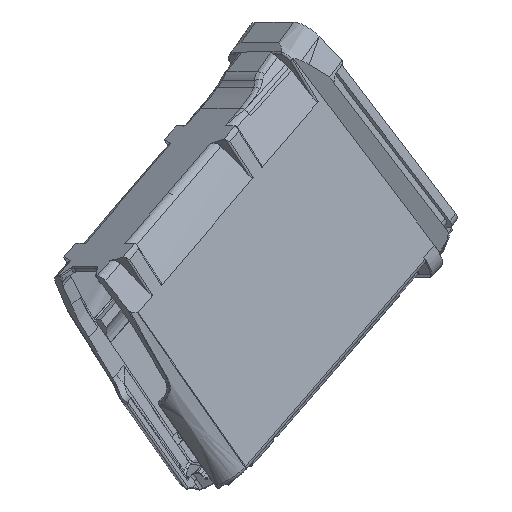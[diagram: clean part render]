
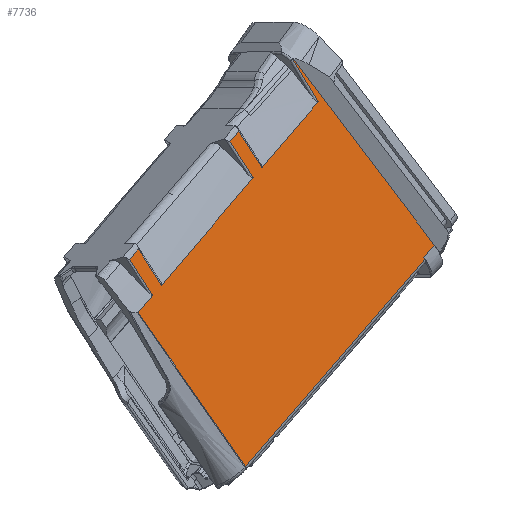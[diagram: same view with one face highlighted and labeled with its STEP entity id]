
A CAD part, top view. The second image highlights one B-rep face of the part: STEP entity #7736.
In plain terms, the highlighted face is planar.
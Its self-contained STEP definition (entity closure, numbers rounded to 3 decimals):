
#90 = EDGE_CURVE ( 'NONE', #14486, #7522, #11005, .T. ) ;
#168 = ORIENTED_EDGE ( 'NONE', *, *, #10661, .F. ) ;
#530 = VERTEX_POINT ( 'NONE', #7717 ) ;
#816 = ORIENTED_EDGE ( 'NONE', *, *, #90, .T. ) ;
#1443 = EDGE_CURVE ( 'NONE', #23993, #14486, #10864, .T. ) ;
#1557 = ORIENTED_EDGE ( 'NONE', *, *, #4731, .F. ) ;
#1852 = VERTEX_POINT ( 'NONE', #3733 ) ;
#2073 = EDGE_CURVE ( 'NONE', #16936, #530, #20423, .T. ) ;
#2199 = ORIENTED_EDGE ( 'NONE', *, *, #11765, .T. ) ;
#2383 = CARTESIAN_POINT ( 'NONE',  ( -29.284, 11.2, 43.909 ) ) ;
#2673 = EDGE_CURVE ( 'NONE', #12823, #11737, #12786, .T. ) ;
#2910 = VECTOR ( 'NONE', #3819, 1000. ) ;
#3134 = ORIENTED_EDGE ( 'NONE', *, *, #4787, .T. ) ;
#3635 = DIRECTION ( 'NONE',  ( -0.766, 0., 0.642 ) ) ;
#3688 = VERTEX_POINT ( 'NONE', #2383 ) ;
#3733 = CARTESIAN_POINT ( 'NONE',  ( 53.633, 11.2, 65.443 ) ) ;
#3819 = DIRECTION ( 'NONE',  ( -0.766, 0., 0.642 ) ) ;
#4002 = CARTESIAN_POINT ( 'NONE',  ( 6.541, 11.2, 99.837 ) ) ;
#4016 = CARTESIAN_POINT ( 'NONE',  ( 18.562, 11.2, 85.202 ) ) ;
#4152 = DIRECTION ( 'NONE',  ( -0.766, 0., 0.642 ) ) ;
#4637 = DIRECTION ( 'NONE',  ( -0.732, 0., -0.682 ) ) ;
#4731 = EDGE_CURVE ( 'NONE', #7395, #26562, #22648, .T. ) ;
#4787 = EDGE_CURVE ( 'NONE', #10811, #17255, #15645, .T. ) ;
#5304 = VECTOR ( 'NONE', #20542, 1000. ) ;
#5463 = DIRECTION ( 'NONE',  ( -0.664, 0., -0.748 ) ) ;
#6243 = CARTESIAN_POINT ( 'NONE',  ( -28.739, 11.2, 60.549 ) ) ;
#6341 = LINE ( 'NONE', #12766, #2910 ) ;
#6432 = DIRECTION ( 'NONE',  ( 0.642, 0., 0.766 ) ) ;
#7179 = DIRECTION ( 'NONE',  ( 0.668, 0., 0.744 ) ) ;
#7395 = VERTEX_POINT ( 'NONE', #25518 ) ;
#7498 = CARTESIAN_POINT ( 'NONE',  ( -28.949, 11.2, 44.282 ) ) ;
#7522 = VERTEX_POINT ( 'NONE', #4002 ) ;
#7529 = ORIENTED_EDGE ( 'NONE', *, *, #29521, .F. ) ;
#7671 = CARTESIAN_POINT ( 'NONE',  ( -39.125, 11.2, 51.369 ) ) ;
#7717 = CARTESIAN_POINT ( 'NONE',  ( -22.535, 11.2, 67.458 ) ) ;
#7736 = ADVANCED_FACE ( 'NONE', ( #12727 ), #21843, .T. ) ;
#7946 = CARTESIAN_POINT ( 'NONE',  ( 10.178, 11.2, 7.584 ) ) ;
#8231 = LINE ( 'NONE', #13313, #20940 ) ;
#8655 = VECTOR ( 'NONE', #13233, 1000. ) ;
#8892 = CARTESIAN_POINT ( 'NONE',  ( 3.22, 11.2, 9.402 ) ) ;
#9226 = EDGE_LOOP ( 'NONE', ( #9680, #25119, #14681, #28991, #9619, #1557, #20260, #24304, #816, #7529, #3134, #14672, #2199, #14942, #24075, #168 ) ) ;
#9426 = CARTESIAN_POINT ( 'NONE',  ( 18.694, 11.2, 97.338 ) ) ;
#9619 = ORIENTED_EDGE ( 'NONE', *, *, #10524, .T. ) ;
#9653 = VECTOR ( 'NONE', #7179, 1000. ) ;
#9680 = ORIENTED_EDGE ( 'NONE', *, *, #16554, .F. ) ;
#10090 = VECTOR ( 'NONE', #3635, 1000. ) ;
#10524 = EDGE_CURVE ( 'NONE', #530, #26562, #29229, .T. ) ;
#10661 = EDGE_CURVE ( 'NONE', #22935, #12787, #11903, .T. ) ;
#10811 = VERTEX_POINT ( 'NONE', #14412 ) ;
#10864 = LINE ( 'NONE', #4016, #10090 ) ;
#11005 = LINE ( 'NONE', #24610, #13887 ) ;
#11281 = EDGE_CURVE ( 'NONE', #3688, #16936, #14678, .T. ) ;
#11395 = EDGE_CURVE ( 'NONE', #12787, #12823, #8231, .T. ) ;
#11601 = DIRECTION ( 'NONE',  ( 0.668, 0., 0.744 ) ) ;
#11737 = VERTEX_POINT ( 'NONE', #14265 ) ;
#11765 = EDGE_CURVE ( 'NONE', #1852, #11737, #24121, .T. ) ;
#11903 = LINE ( 'NONE', #28015, #12302 ) ;
#12019 = VERTEX_POINT ( 'NONE', #27665 ) ;
#12302 = VECTOR ( 'NONE', #16693, 1000. ) ;
#12574 = DIRECTION ( 'NONE',  ( 0.668, 0., 0.744 ) ) ;
#12610 = CARTESIAN_POINT ( 'NONE',  ( 5.777, 11.2, 11.488 ) ) ;
#12727 = FACE_OUTER_BOUND ( 'NONE', #9226, .T. ) ;
#12766 = CARTESIAN_POINT ( 'NONE',  ( 20.897, 11.2, 87.802 ) ) ;
#12786 = LINE ( 'NONE', #27098, #8655 ) ;
#12787 = VERTEX_POINT ( 'NONE', #8892 ) ;
#12823 = VERTEX_POINT ( 'NONE', #17882 ) ;
#13103 = CARTESIAN_POINT ( 'NONE',  ( -28.949, 11.2, 44.282 ) ) ;
#13233 = DIRECTION ( 'NONE',  ( 0.739, 0., -0.674 ) ) ;
#13313 = CARTESIAN_POINT ( 'NONE',  ( 3.096, 11.2, 9.255 ) ) ;
#13551 = CARTESIAN_POINT ( 'NONE',  ( -5.844, 11.2, 58.023 ) ) ;
#13887 = VECTOR ( 'NONE', #11601, 1000. ) ;
#13931 = VECTOR ( 'NONE', #4637, 1000. ) ;
#14265 = CARTESIAN_POINT ( 'NONE',  ( 6.467, 11.2, 12.265 ) ) ;
#14412 = CARTESIAN_POINT ( 'NONE',  ( 14.755, 11.2, 92.951 ) ) ;
#14416 = VECTOR ( 'NONE', #15928, 1000. ) ;
#14486 = VERTEX_POINT ( 'NONE', #16905 ) ;
#14672 = ORIENTED_EDGE ( 'NONE', *, *, #14871, .T. ) ;
#14678 = LINE ( 'NONE', #7498, #20896 ) ;
#14681 = ORIENTED_EDGE ( 'NONE', *, *, #11281, .T. ) ;
#14871 = EDGE_CURVE ( 'NONE', #17255, #1852, #16826, .T. ) ;
#14879 = CARTESIAN_POINT ( 'NONE',  ( 53.632, 11.2, 65.444 ) ) ;
#14942 = ORIENTED_EDGE ( 'NONE', *, *, #2673, .F. ) ;
#15307 = VECTOR ( 'NONE', #5463, 1000. ) ;
#15645 = LINE ( 'NONE', #13103, #5304 ) ;
#15928 = DIRECTION ( 'NONE',  ( 0.789, 0., -0.614 ) ) ;
#16554 = EDGE_CURVE ( 'NONE', #12019, #22935, #25089, .T. ) ;
#16693 = DIRECTION ( 'NONE',  ( 0.71, 0., -0.704 ) ) ;
#16826 = LINE ( 'NONE', #14879, #29156 ) ;
#16905 = CARTESIAN_POINT ( 'NONE',  ( 4.206, 11.2, 97.237 ) ) ;
#16936 = VERTEX_POINT ( 'NONE', #24254 ) ;
#17083 = DIRECTION ( 'NONE',  ( -0.766, 0., 0.642 ) ) ;
#17255 = VERTEX_POINT ( 'NONE', #9426 ) ;
#17297 = EDGE_CURVE ( 'NONE', #7395, #23993, #18550, .T. ) ;
#17882 = CARTESIAN_POINT ( 'NONE',  ( 5.987, 11.2, 12.703 ) ) ;
#18152 = LINE ( 'NONE', #29043, #14416 ) ;
#18550 = LINE ( 'NONE', #27650, #9653 ) ;
#18596 = CARTESIAN_POINT ( 'NONE',  ( 12.42, 11.2, 90.351 ) ) ;
#18652 = CARTESIAN_POINT ( 'NONE',  ( -38.147, 11.2, 52.28 ) ) ;
#18662 = VECTOR ( 'NONE', #24332, 1000. ) ;
#20260 = ORIENTED_EDGE ( 'NONE', *, *, #17297, .T. ) ;
#20423 = LINE ( 'NONE', #22526, #18662 ) ;
#20542 = DIRECTION ( 'NONE',  ( 0.668, 0., 0.744 ) ) ;
#20896 = VECTOR ( 'NONE', #12574, 1000. ) ;
#20940 = VECTOR ( 'NONE', #6432, 1000. ) ;
#21502 = VECTOR ( 'NONE', #4152, 1000. ) ;
#21843 = PLANE ( 'NONE',  #26569 ) ;
#22046 = EDGE_CURVE ( 'NONE', #12019, #3688, #18152, .T. ) ;
#22526 = CARTESIAN_POINT ( 'NONE',  ( -8.178, 11.2, 55.423 ) ) ;
#22648 = LINE ( 'NONE', #13551, #21502 ) ;
#22935 = VERTEX_POINT ( 'NONE', #7671 ) ;
#23787 = DIRECTION ( 'NONE',  ( 0., 1., 0. ) ) ;
#23920 = CARTESIAN_POINT ( 'NONE',  ( -20.2, 11.2, 70.058 ) ) ;
#23993 = VERTEX_POINT ( 'NONE', #18596 ) ;
#24075 = ORIENTED_EDGE ( 'NONE', *, *, #11395, .F. ) ;
#24121 = LINE ( 'NONE', #12610, #15307 ) ;
#24254 = CARTESIAN_POINT ( 'NONE',  ( -14.321, 11.2, 60.572 ) ) ;
#24304 = ORIENTED_EDGE ( 'NONE', *, *, #1443, .T. ) ;
#24332 = DIRECTION ( 'NONE',  ( -0.766, 0., 0.642 ) ) ;
#24610 = CARTESIAN_POINT ( 'NONE',  ( -28.739, 11.2, 60.549 ) ) ;
#25089 = LINE ( 'NONE', #18652, #13931 ) ;
#25119 = ORIENTED_EDGE ( 'NONE', *, *, #22046, .T. ) ;
#25518 = CARTESIAN_POINT ( 'NONE',  ( -11.986, 11.2, 63.172 ) ) ;
#26562 = VERTEX_POINT ( 'NONE', #23920 ) ;
#26569 = AXIS2_PLACEMENT_3D ( 'NONE', #7946, #23787, #17083 ) ;
#27098 = CARTESIAN_POINT ( 'NONE',  ( 7.634, 11.2, 11.199 ) ) ;
#27650 = CARTESIAN_POINT ( 'NONE',  ( -28.949, 11.2, 44.282 ) ) ;
#27665 = CARTESIAN_POINT ( 'NONE',  ( -39.01, 11.2, 51.476 ) ) ;
#28015 = CARTESIAN_POINT ( 'NONE',  ( 7.639, 11.2, 5.022 ) ) ;
#28049 = VECTOR ( 'NONE', #29531, 1000. ) ;
#28140 = DIRECTION ( 'NONE',  ( 0.739, 0., -0.674 ) ) ;
#28991 = ORIENTED_EDGE ( 'NONE', *, *, #2073, .T. ) ;
#29043 = CARTESIAN_POINT ( 'NONE',  ( 12.904, 11.2, 11.088 ) ) ;
#29156 = VECTOR ( 'NONE', #28140, 1000. ) ;
#29229 = LINE ( 'NONE', #6243, #28049 ) ;
#29521 = EDGE_CURVE ( 'NONE', #10811, #7522, #6341, .T. ) ;
#29531 = DIRECTION ( 'NONE',  ( 0.668, 0., 0.744 ) ) ;
